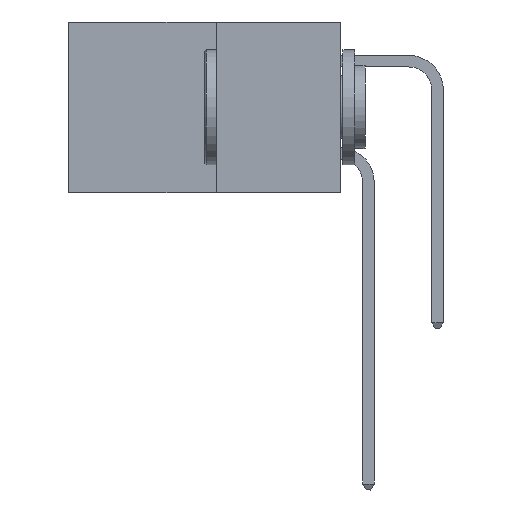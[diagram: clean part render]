
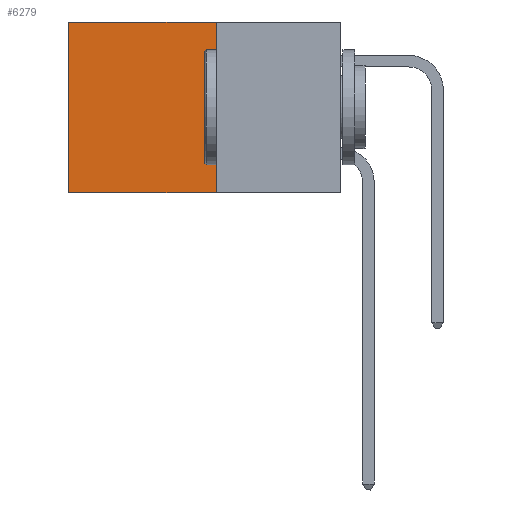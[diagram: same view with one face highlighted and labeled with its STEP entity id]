
A CAD part, left-side view. The second image highlights one B-rep face of the part: STEP entity #6279.
In plain terms, the highlighted planar face has unit normal (-1, 0, 0).
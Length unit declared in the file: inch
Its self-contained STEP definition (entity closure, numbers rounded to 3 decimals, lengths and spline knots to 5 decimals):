
#289 = ORIENTED_EDGE ( 'NONE', *, *, #14955, .F. ) ;
#329 = CARTESIAN_POINT ( 'NONE',  ( 0.277, 0.27, -0.37 ) ) ;
#829 = LINE ( 'NONE', #11095, #9839 ) ;
#1202 = ORIENTED_EDGE ( 'NONE', *, *, #9383, .T. ) ;
#1536 = PLANE ( 'NONE',  #1654 ) ;
#1557 = VECTOR ( 'NONE', #13501, 39.37008 ) ;
#1654 = AXIS2_PLACEMENT_3D ( 'NONE', #329, #10885, #3854 ) ;
#2134 = FACE_OUTER_BOUND ( 'NONE', #8307, .T. ) ;
#3418 = LINE ( 'NONE', #4553, #3769 ) ;
#3769 = VECTOR ( 'NONE', #12696, 39.37008 ) ;
#3770 = CARTESIAN_POINT ( 'NONE',  ( 0.277, 0.27, 0. ) ) ;
#3854 = DIRECTION ( 'NONE',  ( 0., 0., -1. ) ) ;
#4553 = CARTESIAN_POINT ( 'NONE',  ( 0.277, 0.59, -0.37 ) ) ;
#4963 = LINE ( 'NONE', #11493, #13807 ) ;
#5120 = CARTESIAN_POINT ( 'NONE',  ( 0.277, 0.59, 0. ) ) ;
#5900 = ORIENTED_EDGE ( 'NONE', *, *, #13150, .F. ) ;
#6279 = ADVANCED_FACE ( 'NONE', ( #2134 ), #1536, .F. ) ;
#6731 = VERTEX_POINT ( 'NONE', #13799 ) ;
#7617 = VERTEX_POINT ( 'NONE', #3770 ) ;
#8307 = EDGE_LOOP ( 'NONE', ( #1202, #289, #5900, #14180 ) ) ;
#8588 = VERTEX_POINT ( 'NONE', #14733 ) ;
#8906 = LINE ( 'NONE', #12398, #1557 ) ;
#9037 = VERTEX_POINT ( 'NONE', #5120 ) ;
#9383 = EDGE_CURVE ( 'NONE', #9037, #8588, #3418, .T. ) ;
#9839 = VECTOR ( 'NONE', #12227, 39.37008 ) ;
#10885 = DIRECTION ( 'NONE',  ( 1., 0., 0. ) ) ;
#11095 = CARTESIAN_POINT ( 'NONE',  ( 0.277, 0.27, -0.37 ) ) ;
#11493 = CARTESIAN_POINT ( 'NONE',  ( 0.277, 0.27, -0.37 ) ) ;
#11897 = EDGE_CURVE ( 'NONE', #7617, #9037, #8906, .T. ) ;
#12227 = DIRECTION ( 'NONE',  ( 0., 1., 0. ) ) ;
#12398 = CARTESIAN_POINT ( 'NONE',  ( 0.277, 0.27, 0. ) ) ;
#12614 = DIRECTION ( 'NONE',  ( 0., 0., -1. ) ) ;
#12696 = DIRECTION ( 'NONE',  ( 0., 0., -1. ) ) ;
#13150 = EDGE_CURVE ( 'NONE', #7617, #6731, #4963, .T. ) ;
#13501 = DIRECTION ( 'NONE',  ( 0., 1., 0. ) ) ;
#13799 = CARTESIAN_POINT ( 'NONE',  ( 0.277, 0.27, -0.37 ) ) ;
#13807 = VECTOR ( 'NONE', #12614, 39.37008 ) ;
#14180 = ORIENTED_EDGE ( 'NONE', *, *, #11897, .T. ) ;
#14733 = CARTESIAN_POINT ( 'NONE',  ( 0.277, 0.59, -0.37 ) ) ;
#14955 = EDGE_CURVE ( 'NONE', #6731, #8588, #829, .T. ) ;
